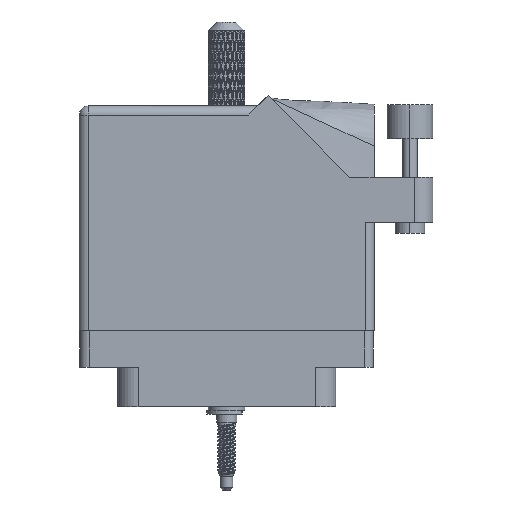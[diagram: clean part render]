
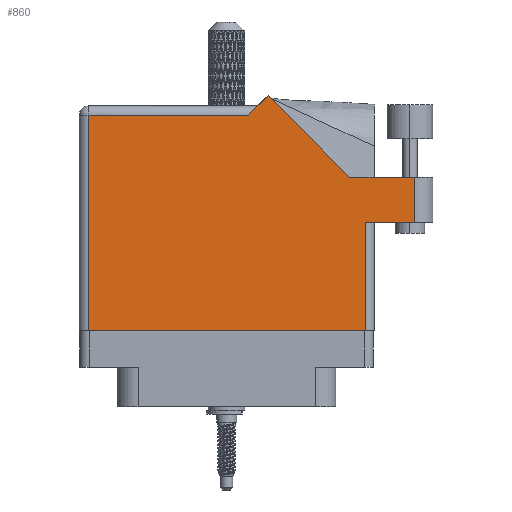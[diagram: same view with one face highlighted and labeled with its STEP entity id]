
A CAD part, front view. The second image highlights one B-rep face of the part: STEP entity #860.
In plain terms, the highlighted face is planar.
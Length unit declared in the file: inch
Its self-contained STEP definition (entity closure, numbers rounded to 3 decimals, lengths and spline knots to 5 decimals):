
#860 = ADVANCED_FACE ( 'NONE', ( #68772 ), #64800, .F. ) ;
#3132 = AXIS2_PLACEMENT_3D ( 'NONE', #24083, #81185, #89393 ) ;
#4317 = CARTESIAN_POINT ( 'NONE',  ( 0.943, 0.637, 0.455 ) ) ;
#5135 = EDGE_CURVE ( 'NONE', #101453, #84578, #69474, .T. ) ;
#7217 = CARTESIAN_POINT ( 'NONE',  ( 0.212, 1.43, 0.455 ) ) ;
#11164 = CARTESIAN_POINT ( 'NONE',  ( 1.005, 0.637, 0.455 ) ) ;
#11366 = VECTOR ( 'NONE', #79980, 39.37008 ) ;
#14875 = ORIENTED_EDGE ( 'NONE', *, *, #42438, .T. ) ;
#16048 = CARTESIAN_POINT ( 'NONE',  ( -1.005, -0.1, 0.455 ) ) ;
#17585 = ORIENTED_EDGE ( 'NONE', *, *, #30476, .T. ) ;
#18068 = ORIENTED_EDGE ( 'NONE', *, *, #45988, .T. ) ;
#18324 = VECTOR ( 'NONE', #61156, 39.37008 ) ;
#20481 = VECTOR ( 'NONE', #31735, 39.37008 ) ;
#22925 = CARTESIAN_POINT ( 'NONE',  ( 1.405, 0.944, 0.455 ) ) ;
#24083 = CARTESIAN_POINT ( 'NONE',  ( -1.005, 1.43, 0.455 ) ) ;
#25591 = CARTESIAN_POINT ( 'NONE',  ( 0.943, -0.1, 0.455 ) ) ;
#26783 = DIRECTION ( 'NONE',  ( 1., 0., 0. ) ) ;
#26841 = VERTEX_POINT ( 'NONE', #25591 ) ;
#30476 = EDGE_CURVE ( 'NONE', #69540, #103419, #88906, .T. ) ;
#31735 = DIRECTION ( 'NONE',  ( 1., 0., 0. ) ) ;
#33178 = ORIENTED_EDGE ( 'NONE', *, *, #44897, .T. ) ;
#34521 = LINE ( 'NONE', #11164, #75272 ) ;
#37164 = VECTOR ( 'NONE', #67700, 39.37008 ) ;
#37987 = CARTESIAN_POINT ( 'NONE',  ( -1.005, 1.368, 0.455 ) ) ;
#42438 = EDGE_CURVE ( 'NONE', #84578, #77628, #47461, .T. ) ;
#42677 = CARTESIAN_POINT ( 'NONE',  ( 0.28271, 1.50071, 0.455 ) ) ;
#43308 = LINE ( 'NONE', #22925, #11366 ) ;
#43773 = CARTESIAN_POINT ( 'NONE',  ( 0.83942, 0.944, 0.455 ) ) ;
#44897 = EDGE_CURVE ( 'NONE', #104888, #69540, #34521, .T. ) ;
#45075 = LINE ( 'NONE', #68558, #64157 ) ;
#45388 = DIRECTION ( 'NONE',  ( 0., 1., 0. ) ) ;
#45988 = EDGE_CURVE ( 'NONE', #103419, #101453, #43308, .T. ) ;
#47461 = LINE ( 'NONE', #7217, #37164 ) ;
#49212 = CARTESIAN_POINT ( 'NONE',  ( -0.943, 1.368, 0.455 ) ) ;
#51499 = DIRECTION ( 'NONE',  ( 0., -1., 0. ) ) ;
#56886 = CARTESIAN_POINT ( 'NONE',  ( 1.28, 0.944, 0.455 ) ) ;
#56955 = ORIENTED_EDGE ( 'NONE', *, *, #84014, .T. ) ;
#57683 = EDGE_CURVE ( 'NONE', #77628, #59509, #61694, .T. ) ;
#59509 = VERTEX_POINT ( 'NONE', #49212 ) ;
#61156 = DIRECTION ( 'NONE',  ( -1., 0., 0. ) ) ;
#61694 = LINE ( 'NONE', #37987, #18324 ) ;
#62150 = ORIENTED_EDGE ( 'NONE', *, *, #57683, .T. ) ;
#64157 = VECTOR ( 'NONE', #51499, 39.37008 ) ;
#64800 = PLANE ( 'NONE',  #3132 ) ;
#67700 = DIRECTION ( 'NONE',  ( -0.707, -0.707, 0. ) ) ;
#68558 = CARTESIAN_POINT ( 'NONE',  ( -0.943, -0.1, 0.455 ) ) ;
#68772 = FACE_OUTER_BOUND ( 'NONE', #87102, .T. ) ;
#69308 = VECTOR ( 'NONE', #45388, 39.37008 ) ;
#69474 = LINE ( 'NONE', #43773, #87362 ) ;
#69540 = VERTEX_POINT ( 'NONE', #100079 ) ;
#69729 = CARTESIAN_POINT ( 'NONE',  ( -0.943, -0.1, 0.455 ) ) ;
#73219 = DIRECTION ( 'NONE',  ( 0., 1., 0. ) ) ;
#73548 = VECTOR ( 'NONE', #73219, 39.37008 ) ;
#75272 = VECTOR ( 'NONE', #26783, 39.37008 ) ;
#75447 = VERTEX_POINT ( 'NONE', #69729 ) ;
#76541 = CARTESIAN_POINT ( 'NONE',  ( 0.943, 0.637, 0.455 ) ) ;
#77628 = VERTEX_POINT ( 'NONE', #80494 ) ;
#77707 = ORIENTED_EDGE ( 'NONE', *, *, #5135, .T. ) ;
#79980 = DIRECTION ( 'NONE',  ( -1., 0., 0. ) ) ;
#80494 = CARTESIAN_POINT ( 'NONE',  ( 0.15, 1.368, 0.455 ) ) ;
#81185 = DIRECTION ( 'NONE',  ( 0., 0., -1. ) ) ;
#82325 = CARTESIAN_POINT ( 'NONE',  ( 0.83942, 0.944, 0.455 ) ) ;
#84014 = EDGE_CURVE ( 'NONE', #75447, #26841, #98383, .T. ) ;
#84491 = ORIENTED_EDGE ( 'NONE', *, *, #90613, .T. ) ;
#84578 = VERTEX_POINT ( 'NONE', #42677 ) ;
#87102 = EDGE_LOOP ( 'NONE', ( #33178, #17585, #18068, #77707, #14875, #62150, #84491, #56955, #94375 ) ) ;
#87362 = VECTOR ( 'NONE', #99485, 39.37008 ) ;
#88906 = LINE ( 'NONE', #56886, #73548 ) ;
#89393 = DIRECTION ( 'NONE',  ( -1., 0., 0. ) ) ;
#90613 = EDGE_CURVE ( 'NONE', #59509, #75447, #45075, .T. ) ;
#91693 = EDGE_CURVE ( 'NONE', #26841, #104888, #101277, .T. ) ;
#94375 = ORIENTED_EDGE ( 'NONE', *, *, #91693, .T. ) ;
#98383 = LINE ( 'NONE', #16048, #20481 ) ;
#99485 = DIRECTION ( 'NONE',  ( -0.707, 0.707, 0. ) ) ;
#99495 = CARTESIAN_POINT ( 'NONE',  ( 1.28, 0.944, 0.455 ) ) ;
#100079 = CARTESIAN_POINT ( 'NONE',  ( 1.28, 0.637, 0.455 ) ) ;
#101277 = LINE ( 'NONE', #4317, #69308 ) ;
#101453 = VERTEX_POINT ( 'NONE', #82325 ) ;
#103419 = VERTEX_POINT ( 'NONE', #99495 ) ;
#104888 = VERTEX_POINT ( 'NONE', #76541 ) ;
